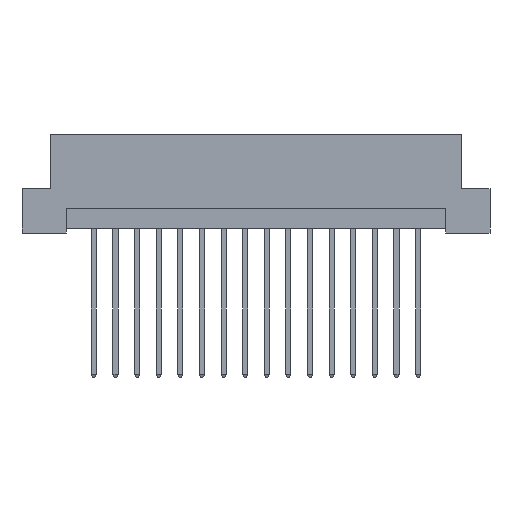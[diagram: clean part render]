
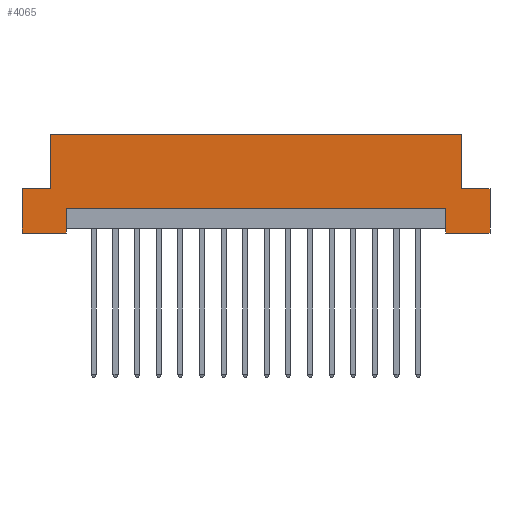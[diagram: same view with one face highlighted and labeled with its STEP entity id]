
A CAD part, front view. The second image highlights one B-rep face of the part: STEP entity #4065.
In plain terms, the highlighted planar face has unit normal (0, -1, 0).
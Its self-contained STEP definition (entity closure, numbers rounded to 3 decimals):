
#53 = VECTOR ( 'NONE', #7478, 1000. ) ;
#121 = VECTOR ( 'NONE', #2136, 1000. ) ;
#185 = ORIENTED_EDGE ( 'NONE', *, *, #3613, .F. ) ;
#460 = DIRECTION ( 'NONE',  ( 0., 0., 1. ) ) ;
#845 = VERTEX_POINT ( 'NONE', #1019 ) ;
#905 = LINE ( 'NONE', #4625, #53 ) ;
#1019 = CARTESIAN_POINT ( 'NONE',  ( 24.2, 0., 5.2 ) ) ;
#1233 = CARTESIAN_POINT ( 'NONE',  ( 27.5, 0., 5.2 ) ) ;
#1373 = CARTESIAN_POINT ( 'NONE',  ( 22.3, 0., 2.9 ) ) ;
#1385 = CARTESIAN_POINT ( 'NONE',  ( -27.5, 0., 0. ) ) ;
#1387 = VERTEX_POINT ( 'NONE', #3307 ) ;
#1500 = VECTOR ( 'NONE', #2046, 1000. ) ;
#1612 = DIRECTION ( 'NONE',  ( 0., 0., -1. ) ) ;
#1718 = LINE ( 'NONE', #5352, #6242 ) ;
#1738 = LINE ( 'NONE', #3843, #4730 ) ;
#1814 = VERTEX_POINT ( 'NONE', #6981 ) ;
#1830 = EDGE_CURVE ( 'NONE', #2954, #1387, #6848, .T. ) ;
#2021 = ORIENTED_EDGE ( 'NONE', *, *, #7400, .T. ) ;
#2046 = DIRECTION ( 'NONE',  ( 0., 0., -1. ) ) ;
#2136 = DIRECTION ( 'NONE',  ( 0., 0., 1. ) ) ;
#2306 = VECTOR ( 'NONE', #4094, 1000. ) ;
#2373 = CARTESIAN_POINT ( 'NONE',  ( -27.5, 0., 11.6 ) ) ;
#2377 = ORIENTED_EDGE ( 'NONE', *, *, #5743, .F. ) ;
#2508 = EDGE_LOOP ( 'NONE', ( #7360, #3047, #6350, #185, #3699, #2021, #6481, #6043, #8050, #5536, #2377, #8536 ) ) ;
#2518 = LINE ( 'NONE', #2373, #7598 ) ;
#2767 = VECTOR ( 'NONE', #9072, 1000. ) ;
#2893 = LINE ( 'NONE', #7820, #1500 ) ;
#2954 = VERTEX_POINT ( 'NONE', #5900 ) ;
#3047 = ORIENTED_EDGE ( 'NONE', *, *, #6370, .T. ) ;
#3171 = DIRECTION ( 'NONE',  ( 1., 0., 0. ) ) ;
#3245 = CARTESIAN_POINT ( 'NONE',  ( -24.2, 0., 5.2 ) ) ;
#3307 = CARTESIAN_POINT ( 'NONE',  ( -24.2, 0., 5.2 ) ) ;
#3331 = CARTESIAN_POINT ( 'NONE',  ( 22.3, 0., 0.5 ) ) ;
#3355 = VECTOR ( 'NONE', #1612, 1000. ) ;
#3437 = DIRECTION ( 'NONE',  ( 0., 0., 1. ) ) ;
#3479 = CARTESIAN_POINT ( 'NONE',  ( 22.3, 0., 0. ) ) ;
#3613 = EDGE_CURVE ( 'NONE', #6874, #6447, #2893, .T. ) ;
#3699 = ORIENTED_EDGE ( 'NONE', *, *, #6792, .F. ) ;
#3764 = LINE ( 'NONE', #5387, #3355 ) ;
#3843 = CARTESIAN_POINT ( 'NONE',  ( 24.2, 0., 5.2 ) ) ;
#4001 = FACE_OUTER_BOUND ( 'NONE', #2508, .T. ) ;
#4065 = ADVANCED_FACE ( 'NONE', ( #4001 ), #7752, .F. ) ;
#4085 = AXIS2_PLACEMENT_3D ( 'NONE', #8381, #9130, #3437 ) ;
#4094 = DIRECTION ( 'NONE',  ( 1., 0., 0. ) ) ;
#4516 = VERTEX_POINT ( 'NONE', #6893 ) ;
#4625 = CARTESIAN_POINT ( 'NONE',  ( -27.5, 0., 0. ) ) ;
#4730 = VECTOR ( 'NONE', #5190, 1000. ) ;
#4771 = EDGE_CURVE ( 'NONE', #6447, #7295, #1718, .T. ) ;
#5059 = EDGE_CURVE ( 'NONE', #5338, #1814, #7855, .T. ) ;
#5074 = CARTESIAN_POINT ( 'NONE',  ( 27.5, 0., 0. ) ) ;
#5190 = DIRECTION ( 'NONE',  ( 0., 0., 1. ) ) ;
#5203 = EDGE_CURVE ( 'NONE', #1814, #7918, #3764, .T. ) ;
#5255 = EDGE_CURVE ( 'NONE', #9073, #8770, #2518, .T. ) ;
#5338 = VERTEX_POINT ( 'NONE', #6814 ) ;
#5352 = CARTESIAN_POINT ( 'NONE',  ( -27.5, 0., 0. ) ) ;
#5387 = CARTESIAN_POINT ( 'NONE',  ( -22.3, 0., 0.5 ) ) ;
#5402 = CARTESIAN_POINT ( 'NONE',  ( -22.3, 0., 0. ) ) ;
#5536 = ORIENTED_EDGE ( 'NONE', *, *, #8695, .F. ) ;
#5743 = EDGE_CURVE ( 'NONE', #7918, #4516, #905, .T. ) ;
#5900 = CARTESIAN_POINT ( 'NONE',  ( -27.5, 0., 5.2 ) ) ;
#6043 = ORIENTED_EDGE ( 'NONE', *, *, #6297, .F. ) ;
#6242 = VECTOR ( 'NONE', #7397, 1000. ) ;
#6259 = VECTOR ( 'NONE', #460, 1000. ) ;
#6297 = EDGE_CURVE ( 'NONE', #1387, #9073, #6837, .T. ) ;
#6350 = ORIENTED_EDGE ( 'NONE', *, *, #4771, .F. ) ;
#6370 = EDGE_CURVE ( 'NONE', #5338, #7295, #9064, .T. ) ;
#6378 = CARTESIAN_POINT ( 'NONE',  ( 27.5, 0., 5.2 ) ) ;
#6447 = VERTEX_POINT ( 'NONE', #5074 ) ;
#6481 = ORIENTED_EDGE ( 'NONE', *, *, #5255, .F. ) ;
#6681 = CARTESIAN_POINT ( 'NONE',  ( 24.2, 0., 11.6 ) ) ;
#6792 = EDGE_CURVE ( 'NONE', #845, #6874, #7711, .T. ) ;
#6814 = CARTESIAN_POINT ( 'NONE',  ( 22.3, 0., 2.9 ) ) ;
#6837 = LINE ( 'NONE', #3245, #6259 ) ;
#6848 = LINE ( 'NONE', #7613, #2767 ) ;
#6874 = VERTEX_POINT ( 'NONE', #6378 ) ;
#6893 = CARTESIAN_POINT ( 'NONE',  ( -27.5, 0., 0. ) ) ;
#6981 = CARTESIAN_POINT ( 'NONE',  ( -22.3, 0., 2.9 ) ) ;
#7295 = VERTEX_POINT ( 'NONE', #3479 ) ;
#7360 = ORIENTED_EDGE ( 'NONE', *, *, #5059, .F. ) ;
#7397 = DIRECTION ( 'NONE',  ( -1., 0., 0. ) ) ;
#7400 = EDGE_CURVE ( 'NONE', #845, #8770, #1738, .T. ) ;
#7478 = DIRECTION ( 'NONE',  ( -1., 0., 0. ) ) ;
#7598 = VECTOR ( 'NONE', #3171, 1000. ) ;
#7613 = CARTESIAN_POINT ( 'NONE',  ( -27.5, 0., 5.2 ) ) ;
#7711 = LINE ( 'NONE', #1233, #2306 ) ;
#7752 = PLANE ( 'NONE',  #4085 ) ;
#7820 = CARTESIAN_POINT ( 'NONE',  ( 27.5, 0., 0. ) ) ;
#7855 = LINE ( 'NONE', #1373, #9239 ) ;
#7918 = VERTEX_POINT ( 'NONE', #5402 ) ;
#7950 = DIRECTION ( 'NONE',  ( -1., 0., 0. ) ) ;
#8050 = ORIENTED_EDGE ( 'NONE', *, *, #1830, .F. ) ;
#8065 = VECTOR ( 'NONE', #9105, 1000. ) ;
#8381 = CARTESIAN_POINT ( 'NONE',  ( -27.5, 0., 11.6 ) ) ;
#8536 = ORIENTED_EDGE ( 'NONE', *, *, #5203, .F. ) ;
#8626 = LINE ( 'NONE', #1385, #121 ) ;
#8695 = EDGE_CURVE ( 'NONE', #4516, #2954, #8626, .T. ) ;
#8770 = VERTEX_POINT ( 'NONE', #6681 ) ;
#9052 = CARTESIAN_POINT ( 'NONE',  ( -24.2, 0., 11.6 ) ) ;
#9064 = LINE ( 'NONE', #3331, #8065 ) ;
#9072 = DIRECTION ( 'NONE',  ( 1., 0., 0. ) ) ;
#9073 = VERTEX_POINT ( 'NONE', #9052 ) ;
#9105 = DIRECTION ( 'NONE',  ( 0., 0., -1. ) ) ;
#9130 = DIRECTION ( 'NONE',  ( 0., 1., 0. ) ) ;
#9239 = VECTOR ( 'NONE', #7950, 1000. ) ;
